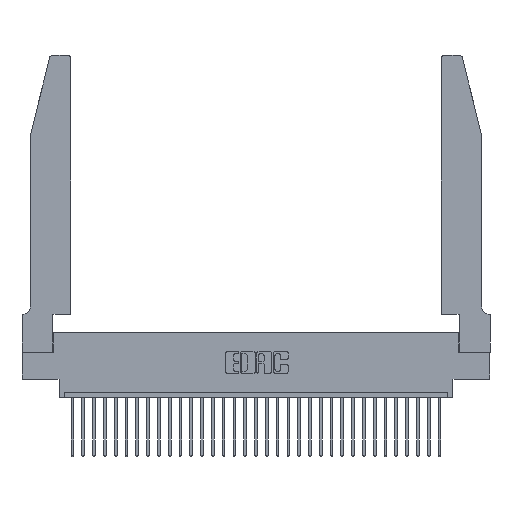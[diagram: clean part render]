
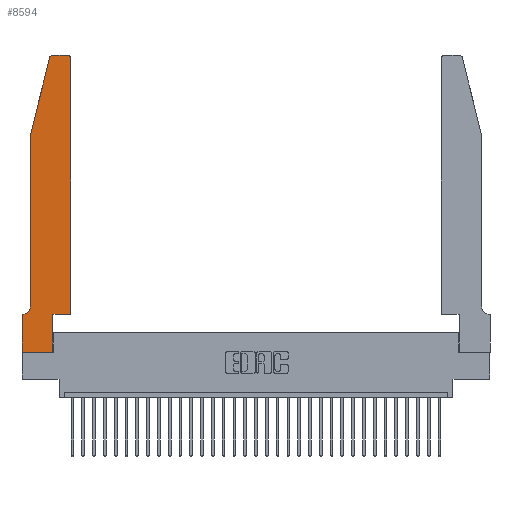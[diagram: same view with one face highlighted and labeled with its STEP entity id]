
A CAD part, top view. The second image highlights one B-rep face of the part: STEP entity #8594.
In plain terms, the highlighted planar face has unit normal (0, 0, 1).
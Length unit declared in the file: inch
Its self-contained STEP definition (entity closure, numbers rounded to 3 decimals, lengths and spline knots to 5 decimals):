
#358 = LINE ( 'NONE', #26154, #17827 ) ;
#623 = ORIENTED_EDGE ( 'NONE', *, *, #4930, .T. ) ;
#1183 = ORIENTED_EDGE ( 'NONE', *, *, #24701, .T. ) ;
#1305 = VERTEX_POINT ( 'NONE', #21911 ) ;
#1550 = DIRECTION ( 'NONE',  ( 0., 0., 1. ) ) ;
#1881 = CARTESIAN_POINT ( 'NONE',  ( 0., 0.35, 0.37 ) ) ;
#2015 = ORIENTED_EDGE ( 'NONE', *, *, #9175, .T. ) ;
#2373 = CARTESIAN_POINT ( 'NONE',  ( 0.0755, 0.42, 0.37 ) ) ;
#2483 = VERTEX_POINT ( 'NONE', #2373 ) ;
#2496 = CARTESIAN_POINT ( 'NONE',  ( 0.2865, 0.35, 0.37 ) ) ;
#2572 = LINE ( 'NONE', #4478, #24376 ) ;
#2908 = CIRCLE ( 'NONE', #15215, 0.07 ) ;
#3255 = DIRECTION ( 'NONE',  ( -0.239, -0.971, 0. ) ) ;
#3780 = AXIS2_PLACEMENT_3D ( 'NONE', #16309, #1550, #29581 ) ;
#4080 = CARTESIAN_POINT ( 'NONE',  ( 0.284, 2.75, 0.37 ) ) ;
#4430 = EDGE_CURVE ( 'NONE', #31472, #30422, #30100, .T. ) ;
#4478 = CARTESIAN_POINT ( 'NONE',  ( 0.0755, 0.35, 0.37 ) ) ;
#4533 = CARTESIAN_POINT ( 'NONE',  ( 0.2865, 0.35, 0.37 ) ) ;
#4795 = CARTESIAN_POINT ( 'NONE',  ( 0.4505, 0.35, 0.37 ) ) ;
#4930 = EDGE_CURVE ( 'NONE', #24192, #25117, #22644, .T. ) ;
#5268 = LINE ( 'NONE', #6218, #20432 ) ;
#6218 = CARTESIAN_POINT ( 'NONE',  ( 0.2605, 2.75, 0.37 ) ) ;
#7358 = DIRECTION ( 'NONE',  ( 1., 0., 0. ) ) ;
#7803 = EDGE_LOOP ( 'NONE', ( #12770, #15036, #22187, #10289, #20020, #23162, #24246, #1183, #2015, #29746, #21414, #623 ) ) ;
#7815 = CARTESIAN_POINT ( 'NONE',  ( 0., 0., 0.37 ) ) ;
#8296 = AXIS2_PLACEMENT_3D ( 'NONE', #17494, #17395, #15197 ) ;
#8399 = CARTESIAN_POINT ( 'NONE',  ( 0.0755, 2., 0.37 ) ) ;
#8517 = DIRECTION ( 'NONE',  ( 0., -1., 0. ) ) ;
#8594 = ADVANCED_FACE ( 'NONE', ( #25207 ), #9002, .T. ) ;
#9002 = PLANE ( 'NONE',  #31497 ) ;
#9175 = EDGE_CURVE ( 'NONE', #15035, #12812, #13885, .T. ) ;
#9285 = CARTESIAN_POINT ( 'NONE',  ( 0.0055, 0.42, 0.37 ) ) ;
#10058 = EDGE_CURVE ( 'NONE', #2483, #28881, #2908, .T. ) ;
#10289 = ORIENTED_EDGE ( 'NONE', *, *, #24205, .T. ) ;
#11033 = EDGE_CURVE ( 'NONE', #30422, #26472, #16098, .T. ) ;
#11481 = DIRECTION ( 'NONE',  ( 0., 0., -1. ) ) ;
#12453 = DIRECTION ( 'NONE',  ( 0., 1., 0. ) ) ;
#12770 = ORIENTED_EDGE ( 'NONE', *, *, #24790, .T. ) ;
#12812 = VERTEX_POINT ( 'NONE', #4533 ) ;
#13885 = LINE ( 'NONE', #2496, #27918 ) ;
#14026 = LINE ( 'NONE', #17385, #18706 ) ;
#14030 = DIRECTION ( 'NONE',  ( 1., 0., 0. ) ) ;
#15035 = VERTEX_POINT ( 'NONE', #23558 ) ;
#15036 = ORIENTED_EDGE ( 'NONE', *, *, #4430, .T. ) ;
#15197 = DIRECTION ( 'NONE',  ( 1., 0., 0. ) ) ;
#15215 = AXIS2_PLACEMENT_3D ( 'NONE', #9285, #11481, #16723 ) ;
#15292 = VECTOR ( 'NONE', #3255, 39.37008 ) ;
#15391 = VERTEX_POINT ( 'NONE', #27744 ) ;
#15868 = CARTESIAN_POINT ( 'NONE',  ( 0.0755, 2., 0.37 ) ) ;
#16098 = LINE ( 'NONE', #15868, #15292 ) ;
#16309 = CARTESIAN_POINT ( 'NONE',  ( 0.284, 2.72, 0.37 ) ) ;
#16723 = DIRECTION ( 'NONE',  ( -1., 0., 0. ) ) ;
#16960 = EDGE_CURVE ( 'NONE', #28881, #1305, #2572, .T. ) ;
#17385 = CARTESIAN_POINT ( 'NONE',  ( 0.4505, 0.35, 0.37 ) ) ;
#17395 = DIRECTION ( 'NONE',  ( 0., 0., 1. ) ) ;
#17494 = CARTESIAN_POINT ( 'NONE',  ( 0.4205, 2.72, 0.37 ) ) ;
#17827 = VECTOR ( 'NONE', #18408, 39.37008 ) ;
#17836 = VERTEX_POINT ( 'NONE', #23232 ) ;
#18197 = EDGE_CURVE ( 'NONE', #12812, #15391, #20745, .T. ) ;
#18408 = DIRECTION ( 'NONE',  ( 0., -1., 0. ) ) ;
#18706 = VECTOR ( 'NONE', #12453, 39.37008 ) ;
#19247 = DIRECTION ( 'NONE',  ( 0., 0., 1. ) ) ;
#20020 = ORIENTED_EDGE ( 'NONE', *, *, #10058, .T. ) ;
#20213 = CARTESIAN_POINT ( 'NONE',  ( 0.4205, 2.75, 0.37 ) ) ;
#20432 = VECTOR ( 'NONE', #30828, 39.37008 ) ;
#20745 = LINE ( 'NONE', #4795, #21518 ) ;
#21210 = LINE ( 'NONE', #7815, #29438 ) ;
#21414 = ORIENTED_EDGE ( 'NONE', *, *, #27842, .T. ) ;
#21518 = VECTOR ( 'NONE', #7358, 39.37008 ) ;
#21911 = CARTESIAN_POINT ( 'NONE',  ( 0., 0.35, 0.37 ) ) ;
#22187 = ORIENTED_EDGE ( 'NONE', *, *, #11033, .T. ) ;
#22498 = CARTESIAN_POINT ( 'NONE',  ( 0.25487, 2.72718, 0.37 ) ) ;
#22552 = EDGE_CURVE ( 'NONE', #1305, #17836, #358, .T. ) ;
#22644 = CIRCLE ( 'NONE', #8296, 0.03 ) ;
#22976 = CARTESIAN_POINT ( 'NONE',  ( 0.0755, 2., 0.37 ) ) ;
#23162 = ORIENTED_EDGE ( 'NONE', *, *, #16960, .T. ) ;
#23232 = CARTESIAN_POINT ( 'NONE',  ( 0., 0., 0.37 ) ) ;
#23558 = CARTESIAN_POINT ( 'NONE',  ( 0.2865, 0., 0.37 ) ) ;
#24192 = VERTEX_POINT ( 'NONE', #25969 ) ;
#24205 = EDGE_CURVE ( 'NONE', #26472, #2483, #25569, .T. ) ;
#24219 = CARTESIAN_POINT ( 'NONE',  ( 0.0055, 0.35, 0.37 ) ) ;
#24246 = ORIENTED_EDGE ( 'NONE', *, *, #22552, .T. ) ;
#24376 = VECTOR ( 'NONE', #26449, 39.37008 ) ;
#24701 = EDGE_CURVE ( 'NONE', #17836, #15035, #21210, .T. ) ;
#24790 = EDGE_CURVE ( 'NONE', #25117, #31472, #5268, .T. ) ;
#24897 = DIRECTION ( 'NONE',  ( 0., 1., 0. ) ) ;
#25117 = VERTEX_POINT ( 'NONE', #20213 ) ;
#25207 = FACE_OUTER_BOUND ( 'NONE', #7803, .T. ) ;
#25569 = LINE ( 'NONE', #8399, #29102 ) ;
#25969 = CARTESIAN_POINT ( 'NONE',  ( 0.4505, 2.72, 0.37 ) ) ;
#26154 = CARTESIAN_POINT ( 'NONE',  ( 0., 0., 0.37 ) ) ;
#26449 = DIRECTION ( 'NONE',  ( -1., 0., 0. ) ) ;
#26472 = VERTEX_POINT ( 'NONE', #22976 ) ;
#27666 = DIRECTION ( 'NONE',  ( 1., 0., 0. ) ) ;
#27744 = CARTESIAN_POINT ( 'NONE',  ( 0.4505, 0.35, 0.37 ) ) ;
#27842 = EDGE_CURVE ( 'NONE', #15391, #24192, #14026, .T. ) ;
#27918 = VECTOR ( 'NONE', #24897, 39.37008 ) ;
#28881 = VERTEX_POINT ( 'NONE', #24219 ) ;
#29102 = VECTOR ( 'NONE', #8517, 39.37008 ) ;
#29438 = VECTOR ( 'NONE', #27666, 39.37008 ) ;
#29581 = DIRECTION ( 'NONE',  ( 1., 0., 0. ) ) ;
#29746 = ORIENTED_EDGE ( 'NONE', *, *, #18197, .T. ) ;
#30100 = CIRCLE ( 'NONE', #3780, 0.03 ) ;
#30422 = VERTEX_POINT ( 'NONE', #22498 ) ;
#30828 = DIRECTION ( 'NONE',  ( -1., 0., 0. ) ) ;
#31472 = VERTEX_POINT ( 'NONE', #4080 ) ;
#31497 = AXIS2_PLACEMENT_3D ( 'NONE', #1881, #19247, #14030 ) ;
